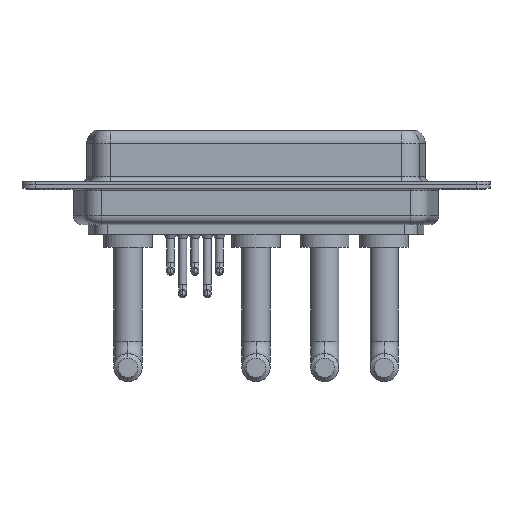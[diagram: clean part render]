
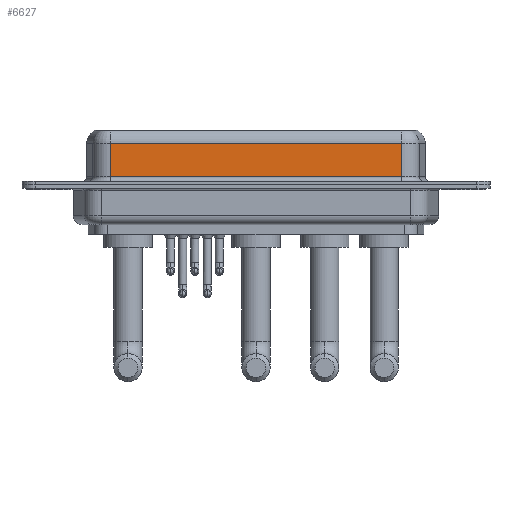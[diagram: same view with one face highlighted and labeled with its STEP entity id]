
A CAD part, front view. The second image highlights one B-rep face of the part: STEP entity #6627.
In plain terms, the highlighted planar face has unit normal (0, -1, 0).
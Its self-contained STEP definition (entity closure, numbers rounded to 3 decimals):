
#54 = LINE ( 'NONE', #12117, #11881 ) ;
#196 = VECTOR ( 'NONE', #5723, 1000. ) ;
#351 = VECTOR ( 'NONE', #7412, 1000. ) ;
#418 = VERTEX_POINT ( 'NONE', #14861 ) ;
#498 = CARTESIAN_POINT ( 'NONE',  ( 40.037, -3.95, 0.9 ) ) ;
#1566 = DIRECTION ( 'NONE',  ( 0., 0., 1. ) ) ;
#1682 = EDGE_CURVE ( 'NONE', #4788, #7044, #14015, .T. ) ;
#2508 = DIRECTION ( 'NONE',  ( -1., 0., 0. ) ) ;
#2736 = PLANE ( 'NONE',  #4405 ) ;
#2882 = ORIENTED_EDGE ( 'NONE', *, *, #5716, .T. ) ;
#3603 = ORIENTED_EDGE ( 'NONE', *, *, #14425, .F. ) ;
#4405 = AXIS2_PLACEMENT_3D ( 'NONE', #7511, #12272, #1566 ) ;
#4788 = VERTEX_POINT ( 'NONE', #11196 ) ;
#5716 = EDGE_CURVE ( 'NONE', #7044, #8452, #14666, .T. ) ;
#5723 = DIRECTION ( 'NONE',  ( 0., 0., -1. ) ) ;
#5946 = CARTESIAN_POINT ( 'NONE',  ( 40.037, -3.95, 0.9 ) ) ;
#6419 = EDGE_CURVE ( 'NONE', #418, #4788, #54, .T. ) ;
#6627 = ADVANCED_FACE ( 'NONE', ( #14611 ), #2736, .F. ) ;
#7044 = VERTEX_POINT ( 'NONE', #11303 ) ;
#7412 = DIRECTION ( 'NONE',  ( 1., 0., 0. ) ) ;
#7511 = CARTESIAN_POINT ( 'NONE',  ( 40.037, -3.95, 6.4 ) ) ;
#7702 = ORIENTED_EDGE ( 'NONE', *, *, #6419, .T. ) ;
#8234 = CARTESIAN_POINT ( 'NONE',  ( 7.013, -3.95, 6.4 ) ) ;
#8452 = VERTEX_POINT ( 'NONE', #5946 ) ;
#8639 = ORIENTED_EDGE ( 'NONE', *, *, #1682, .T. ) ;
#9464 = LINE ( 'NONE', #14222, #14630 ) ;
#11196 = CARTESIAN_POINT ( 'NONE',  ( 7.013, -3.95, 4.65 ) ) ;
#11303 = CARTESIAN_POINT ( 'NONE',  ( 7.013, -3.95, 0.9 ) ) ;
#11881 = VECTOR ( 'NONE', #2508, 1000. ) ;
#12117 = CARTESIAN_POINT ( 'NONE',  ( 40.037, -3.95, 4.65 ) ) ;
#12272 = DIRECTION ( 'NONE',  ( 0., 1., 0. ) ) ;
#13027 = EDGE_LOOP ( 'NONE', ( #3603, #7702, #8639, #2882 ) ) ;
#13054 = DIRECTION ( 'NONE',  ( 0., 0., -1. ) ) ;
#14015 = LINE ( 'NONE', #8234, #196 ) ;
#14222 = CARTESIAN_POINT ( 'NONE',  ( 40.037, -3.95, 6.4 ) ) ;
#14425 = EDGE_CURVE ( 'NONE', #418, #8452, #9464, .T. ) ;
#14611 = FACE_OUTER_BOUND ( 'NONE', #13027, .T. ) ;
#14630 = VECTOR ( 'NONE', #13054, 1000. ) ;
#14666 = LINE ( 'NONE', #498, #351 ) ;
#14861 = CARTESIAN_POINT ( 'NONE',  ( 40.037, -3.95, 4.65 ) ) ;
